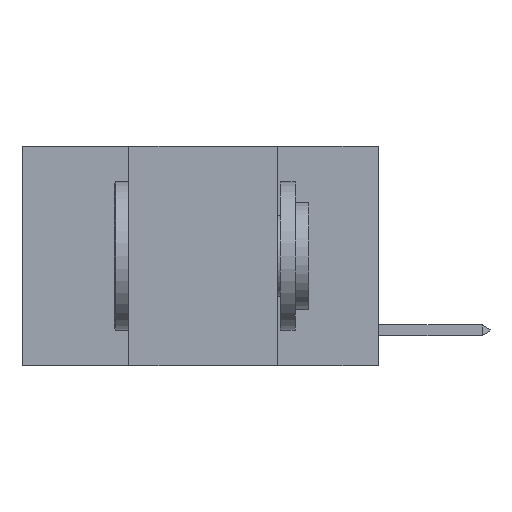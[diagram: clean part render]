
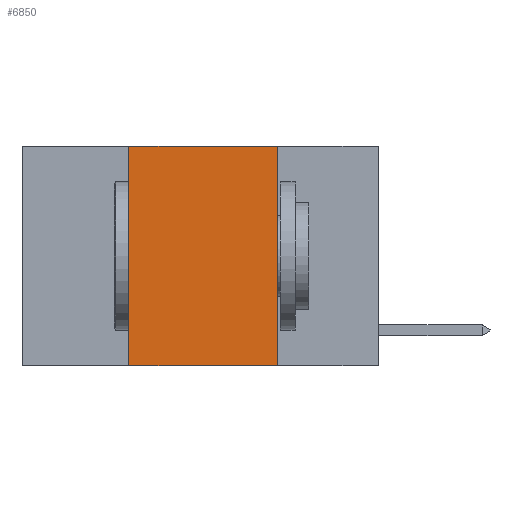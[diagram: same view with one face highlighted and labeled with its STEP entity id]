
A CAD part, left-side view. The second image highlights one B-rep face of the part: STEP entity #6850.
In plain terms, the highlighted planar face has unit normal (-1, 0, 0).
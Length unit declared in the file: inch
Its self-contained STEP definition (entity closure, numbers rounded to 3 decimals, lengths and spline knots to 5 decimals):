
#182 = LINE ( 'NONE', #13560, #9965 ) ;
#405 = ORIENTED_EDGE ( 'NONE', *, *, #5653, .F. ) ;
#624 = EDGE_LOOP ( 'NONE', ( #17370, #16558, #405, #10872 ) ) ;
#1711 = PLANE ( 'NONE',  #10386 ) ;
#3329 = DIRECTION ( 'NONE',  ( 0., 0., -1. ) ) ;
#4956 = EDGE_CURVE ( 'NONE', #11135, #15599, #12353, .T. ) ;
#5115 = VECTOR ( 'NONE', #12502, 39.37008 ) ;
#5532 = EDGE_CURVE ( 'NONE', #12457, #15599, #9498, .T. ) ;
#5653 = EDGE_CURVE ( 'NONE', #11135, #17405, #8847, .T. ) ;
#6079 = CARTESIAN_POINT ( 'NONE',  ( 0., 0.17, -0.37 ) ) ;
#6850 = ADVANCED_FACE ( 'NONE', ( #13416 ), #1711, .F. ) ;
#7328 = DIRECTION ( 'NONE',  ( 0., 0., 1. ) ) ;
#8673 = VECTOR ( 'NONE', #10848, 39.37008 ) ;
#8847 = LINE ( 'NONE', #12848, #15724 ) ;
#9498 = LINE ( 'NONE', #13863, #5115 ) ;
#9965 = VECTOR ( 'NONE', #13621, 39.37008 ) ;
#10073 = CARTESIAN_POINT ( 'NONE',  ( 0., 0.42, -0.37 ) ) ;
#10386 = AXIS2_PLACEMENT_3D ( 'NONE', #10691, #12072, #3329 ) ;
#10691 = CARTESIAN_POINT ( 'NONE',  ( 0., 0.6, 0. ) ) ;
#10848 = DIRECTION ( 'NONE',  ( 0., -1., 0. ) ) ;
#10872 = ORIENTED_EDGE ( 'NONE', *, *, #4956, .T. ) ;
#11135 = VERTEX_POINT ( 'NONE', #10073 ) ;
#12072 = DIRECTION ( 'NONE',  ( 1., 0., 0. ) ) ;
#12353 = LINE ( 'NONE', #16267, #8673 ) ;
#12457 = VERTEX_POINT ( 'NONE', #13760 ) ;
#12502 = DIRECTION ( 'NONE',  ( 0., 0., -1. ) ) ;
#12848 = CARTESIAN_POINT ( 'NONE',  ( 0., 0.42, 0. ) ) ;
#13416 = FACE_OUTER_BOUND ( 'NONE', #624, .T. ) ;
#13560 = CARTESIAN_POINT ( 'NONE',  ( 0., 0.6, 0. ) ) ;
#13621 = DIRECTION ( 'NONE',  ( 0., -1., 0. ) ) ;
#13760 = CARTESIAN_POINT ( 'NONE',  ( 0., 0.17, 0. ) ) ;
#13863 = CARTESIAN_POINT ( 'NONE',  ( 0., 0.17, 0. ) ) ;
#14105 = EDGE_CURVE ( 'NONE', #17405, #12457, #182, .T. ) ;
#15599 = VERTEX_POINT ( 'NONE', #6079 ) ;
#15724 = VECTOR ( 'NONE', #7328, 39.37008 ) ;
#16267 = CARTESIAN_POINT ( 'NONE',  ( 0., 0.6, -0.37 ) ) ;
#16558 = ORIENTED_EDGE ( 'NONE', *, *, #14105, .F. ) ;
#17364 = CARTESIAN_POINT ( 'NONE',  ( 0., 0.42, 0. ) ) ;
#17370 = ORIENTED_EDGE ( 'NONE', *, *, #5532, .F. ) ;
#17405 = VERTEX_POINT ( 'NONE', #17364 ) ;
